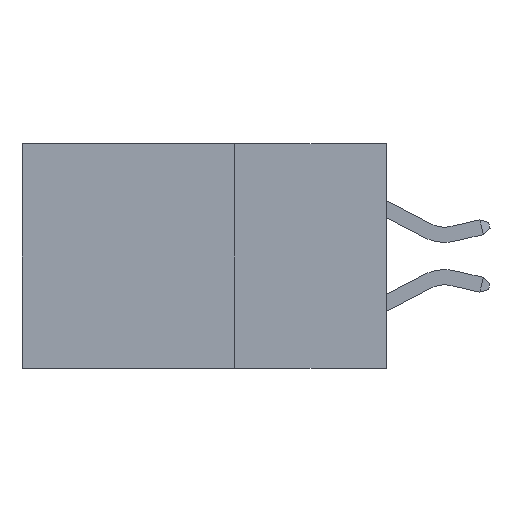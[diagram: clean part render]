
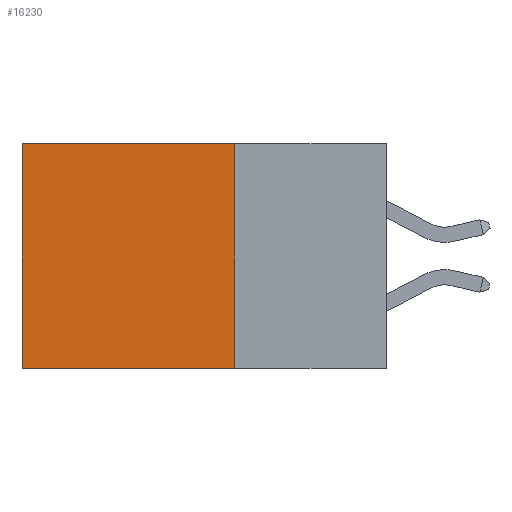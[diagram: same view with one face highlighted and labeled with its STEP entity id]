
A CAD part, left-side view. The second image highlights one B-rep face of the part: STEP entity #16230.
In plain terms, the highlighted planar face has unit normal (-1, 0, 0).
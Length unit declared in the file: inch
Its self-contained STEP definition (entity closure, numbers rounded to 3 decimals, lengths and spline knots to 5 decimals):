
#375 = DIRECTION ( 'NONE',  ( 0., 0., -1. ) ) ;
#1792 = EDGE_CURVE ( 'NONE', #20859, #2095, #19605, .T. ) ;
#1854 = ORIENTED_EDGE ( 'NONE', *, *, #8898, .T. ) ;
#2095 = VERTEX_POINT ( 'NONE', #3885 ) ;
#2531 = VERTEX_POINT ( 'NONE', #13202 ) ;
#3138 = ORIENTED_EDGE ( 'NONE', *, *, #1792, .T. ) ;
#3858 = PLANE ( 'NONE',  #15179 ) ;
#3885 = CARTESIAN_POINT ( 'NONE',  ( 0.2615, 0.6, 0. ) ) ;
#4122 = CARTESIAN_POINT ( 'NONE',  ( 0.2615, 0.6, -0.37 ) ) ;
#5294 = EDGE_CURVE ( 'NONE', #2531, #6865, #23021, .T. ) ;
#6217 = VECTOR ( 'NONE', #15920, 39.37008 ) ;
#6477 = CARTESIAN_POINT ( 'NONE',  ( 0.2615, 0.25, 0. ) ) ;
#6865 = VERTEX_POINT ( 'NONE', #4122 ) ;
#6965 = DIRECTION ( 'NONE',  ( 0., 1., 0. ) ) ;
#7963 = LINE ( 'NONE', #15469, #13597 ) ;
#8898 = EDGE_CURVE ( 'NONE', #2095, #6865, #14398, .T. ) ;
#9260 = DIRECTION ( 'NONE',  ( 0., 0., -1. ) ) ;
#10749 = VECTOR ( 'NONE', #16000, 39.37008 ) ;
#10836 = CARTESIAN_POINT ( 'NONE',  ( 0.2615, 0.6, -0.37 ) ) ;
#11465 = DIRECTION ( 'NONE',  ( 1., 0., 0. ) ) ;
#11926 = ORIENTED_EDGE ( 'NONE', *, *, #13955, .F. ) ;
#12205 = VECTOR ( 'NONE', #6965, 39.37008 ) ;
#13090 = CARTESIAN_POINT ( 'NONE',  ( 0.2615, 0.25, -0.37 ) ) ;
#13202 = CARTESIAN_POINT ( 'NONE',  ( 0.2615, 0.25, -0.37 ) ) ;
#13597 = VECTOR ( 'NONE', #375, 39.37008 ) ;
#13955 = EDGE_CURVE ( 'NONE', #20859, #2531, #7963, .T. ) ;
#14398 = LINE ( 'NONE', #10836, #10749 ) ;
#15179 = AXIS2_PLACEMENT_3D ( 'NONE', #13090, #11465, #9260 ) ;
#15469 = CARTESIAN_POINT ( 'NONE',  ( 0.2615, 0.25, -0.37 ) ) ;
#15920 = DIRECTION ( 'NONE',  ( 0., 1., 0. ) ) ;
#16000 = DIRECTION ( 'NONE',  ( 0., 0., -1. ) ) ;
#16230 = ADVANCED_FACE ( 'NONE', ( #22512 ), #3858, .F. ) ;
#18138 = EDGE_LOOP ( 'NONE', ( #1854, #20232, #11926, #3138 ) ) ;
#19086 = CARTESIAN_POINT ( 'NONE',  ( 0.2615, 0.25, 0. ) ) ;
#19605 = LINE ( 'NONE', #6477, #12205 ) ;
#20232 = ORIENTED_EDGE ( 'NONE', *, *, #5294, .F. ) ;
#20859 = VERTEX_POINT ( 'NONE', #19086 ) ;
#21068 = CARTESIAN_POINT ( 'NONE',  ( 0.2615, 0.25, -0.37 ) ) ;
#22512 = FACE_OUTER_BOUND ( 'NONE', #18138, .T. ) ;
#23021 = LINE ( 'NONE', #21068, #6217 ) ;
